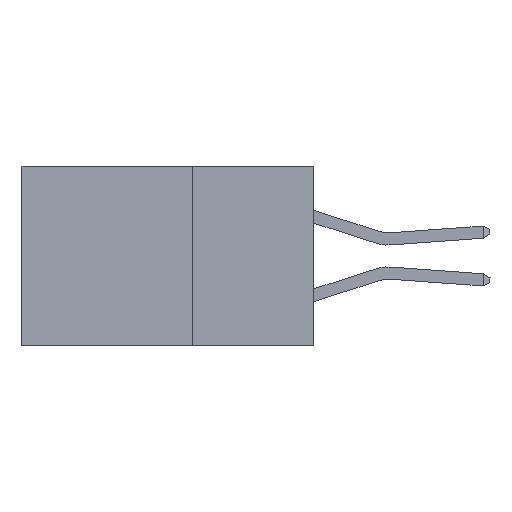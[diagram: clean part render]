
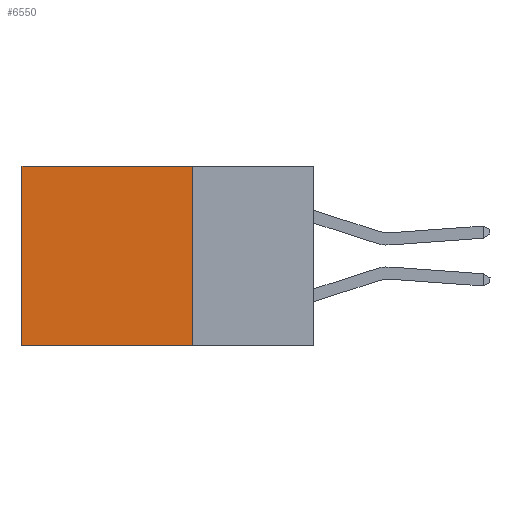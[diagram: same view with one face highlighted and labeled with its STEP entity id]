
A CAD part, left-side view. The second image highlights one B-rep face of the part: STEP entity #6550.
In plain terms, the highlighted planar face has unit normal (-1, 0, 0).
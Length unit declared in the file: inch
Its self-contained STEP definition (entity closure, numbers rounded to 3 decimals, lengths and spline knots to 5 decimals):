
#414 = EDGE_CURVE ( 'NONE', #7358, #3720, #9685, .T. ) ;
#567 = CARTESIAN_POINT ( 'NONE',  ( 0.2875, 0.25, -0.37 ) ) ;
#834 = CARTESIAN_POINT ( 'NONE',  ( 0.2875, 0.6, 0. ) ) ;
#1134 = AXIS2_PLACEMENT_3D ( 'NONE', #6886, #5684, #14393 ) ;
#1152 = CARTESIAN_POINT ( 'NONE',  ( 0.2875, 0.25, 0. ) ) ;
#1871 = CARTESIAN_POINT ( 'NONE',  ( 0.2875, 0.25, -0.37 ) ) ;
#3031 = LINE ( 'NONE', #1871, #14325 ) ;
#3681 = ORIENTED_EDGE ( 'NONE', *, *, #8081, .T. ) ;
#3720 = VERTEX_POINT ( 'NONE', #834 ) ;
#3805 = CARTESIAN_POINT ( 'NONE',  ( 0.2875, 0.6, 0. ) ) ;
#4416 = DIRECTION ( 'NONE',  ( 0., 1., 0. ) ) ;
#4463 = ORIENTED_EDGE ( 'NONE', *, *, #5840, .F. ) ;
#4472 = EDGE_LOOP ( 'NONE', ( #3681, #4463, #7449, #7174 ) ) ;
#5056 = VERTEX_POINT ( 'NONE', #567 ) ;
#5684 = DIRECTION ( 'NONE',  ( 1., 0., 0. ) ) ;
#5840 = EDGE_CURVE ( 'NONE', #5056, #9953, #3031, .T. ) ;
#6550 = ADVANCED_FACE ( 'NONE', ( #14865 ), #13183, .F. ) ;
#6886 = CARTESIAN_POINT ( 'NONE',  ( 0.2875, 0.25, 0. ) ) ;
#7174 = ORIENTED_EDGE ( 'NONE', *, *, #414, .T. ) ;
#7358 = VERTEX_POINT ( 'NONE', #1152 ) ;
#7449 = ORIENTED_EDGE ( 'NONE', *, *, #13875, .F. ) ;
#7770 = VECTOR ( 'NONE', #9899, 39.37008 ) ;
#8081 = EDGE_CURVE ( 'NONE', #3720, #9953, #12534, .T. ) ;
#8667 = CARTESIAN_POINT ( 'NONE',  ( 0.2875, 0.25, 0. ) ) ;
#9305 = VECTOR ( 'NONE', #11890, 39.37008 ) ;
#9685 = LINE ( 'NONE', #11981, #9305 ) ;
#9899 = DIRECTION ( 'NONE',  ( 0., 0., -1. ) ) ;
#9953 = VERTEX_POINT ( 'NONE', #11097 ) ;
#10054 = DIRECTION ( 'NONE',  ( 0., 0., -1. ) ) ;
#11097 = CARTESIAN_POINT ( 'NONE',  ( 0.2875, 0.6, -0.37 ) ) ;
#11890 = DIRECTION ( 'NONE',  ( 0., 1., 0. ) ) ;
#11981 = CARTESIAN_POINT ( 'NONE',  ( 0.2875, 0.25, 0. ) ) ;
#12534 = LINE ( 'NONE', #3805, #15381 ) ;
#13183 = PLANE ( 'NONE',  #1134 ) ;
#13875 = EDGE_CURVE ( 'NONE', #7358, #5056, #13981, .T. ) ;
#13981 = LINE ( 'NONE', #8667, #7770 ) ;
#14325 = VECTOR ( 'NONE', #4416, 39.37008 ) ;
#14393 = DIRECTION ( 'NONE',  ( 0., 0., -1. ) ) ;
#14865 = FACE_OUTER_BOUND ( 'NONE', #4472, .T. ) ;
#15381 = VECTOR ( 'NONE', #10054, 39.37008 ) ;
